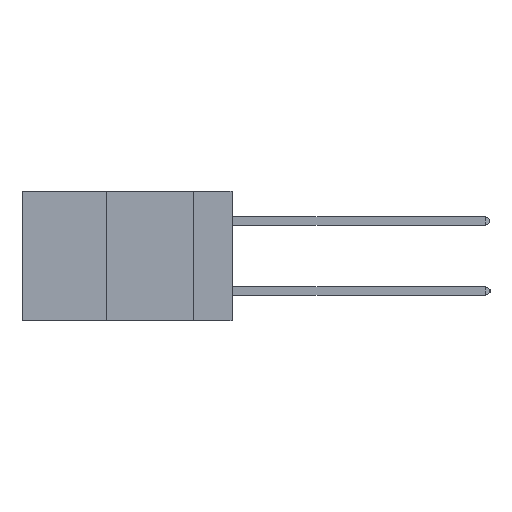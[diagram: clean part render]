
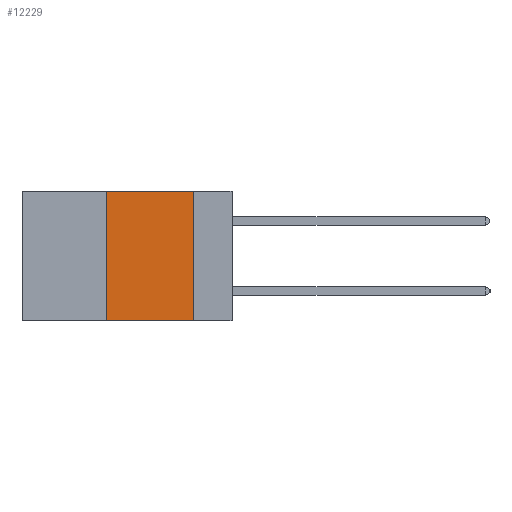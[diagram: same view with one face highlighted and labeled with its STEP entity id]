
A CAD part, left-side view. The second image highlights one B-rep face of the part: STEP entity #12229.
In plain terms, the highlighted planar face has unit normal (-1, 0, 0).
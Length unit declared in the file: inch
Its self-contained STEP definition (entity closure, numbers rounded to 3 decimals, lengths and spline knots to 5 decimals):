
#41 = LINE ( 'NONE', #6378, #4519 ) ;
#276 = VERTEX_POINT ( 'NONE', #10502 ) ;
#443 = VERTEX_POINT ( 'NONE', #11608 ) ;
#1178 = CARTESIAN_POINT ( 'NONE',  ( 0., 0.11, -0.37 ) ) ;
#2066 = CARTESIAN_POINT ( 'NONE',  ( 0., 0.36, 0. ) ) ;
#2390 = DIRECTION ( 'NONE',  ( 0., -1., 0. ) ) ;
#2874 = LINE ( 'NONE', #2066, #11031 ) ;
#3265 = VERTEX_POINT ( 'NONE', #1178 ) ;
#3268 = EDGE_CURVE ( 'NONE', #443, #276, #41, .T. ) ;
#3460 = AXIS2_PLACEMENT_3D ( 'NONE', #5574, #7523, #6670 ) ;
#4008 = EDGE_CURVE ( 'NONE', #11498, #443, #2874, .T. ) ;
#4235 = VECTOR ( 'NONE', #4794, 39.37008 ) ;
#4519 = VECTOR ( 'NONE', #2390, 39.37008 ) ;
#4695 = FACE_OUTER_BOUND ( 'NONE', #4941, .T. ) ;
#4794 = DIRECTION ( 'NONE',  ( 0., -1., 0. ) ) ;
#4941 = EDGE_LOOP ( 'NONE', ( #12663, #9753, #11478, #8268 ) ) ;
#5574 = CARTESIAN_POINT ( 'NONE',  ( 0., 0.6, 0. ) ) ;
#5943 = VECTOR ( 'NONE', #9829, 39.37008 ) ;
#6327 = DIRECTION ( 'NONE',  ( 0., 0., 1. ) ) ;
#6378 = CARTESIAN_POINT ( 'NONE',  ( 0., 0.6, 0. ) ) ;
#6670 = DIRECTION ( 'NONE',  ( 0., 0., -1. ) ) ;
#7146 = CARTESIAN_POINT ( 'NONE',  ( 0., 0.36, -0.37 ) ) ;
#7372 = EDGE_CURVE ( 'NONE', #11498, #3265, #11770, .T. ) ;
#7523 = DIRECTION ( 'NONE',  ( 1., 0., 0. ) ) ;
#7556 = LINE ( 'NONE', #11872, #5943 ) ;
#8268 = ORIENTED_EDGE ( 'NONE', *, *, #7372, .T. ) ;
#9353 = EDGE_CURVE ( 'NONE', #276, #3265, #7556, .T. ) ;
#9753 = ORIENTED_EDGE ( 'NONE', *, *, #3268, .F. ) ;
#9829 = DIRECTION ( 'NONE',  ( 0., 0., -1. ) ) ;
#10502 = CARTESIAN_POINT ( 'NONE',  ( 0., 0.11, 0. ) ) ;
#11031 = VECTOR ( 'NONE', #6327, 39.37008 ) ;
#11034 = CARTESIAN_POINT ( 'NONE',  ( 0., 0.6, -0.37 ) ) ;
#11478 = ORIENTED_EDGE ( 'NONE', *, *, #4008, .F. ) ;
#11498 = VERTEX_POINT ( 'NONE', #7146 ) ;
#11608 = CARTESIAN_POINT ( 'NONE',  ( 0., 0.36, 0. ) ) ;
#11770 = LINE ( 'NONE', #11034, #4235 ) ;
#11872 = CARTESIAN_POINT ( 'NONE',  ( 0., 0.11, 0. ) ) ;
#12229 = ADVANCED_FACE ( 'NONE', ( #4695 ), #12794, .F. ) ;
#12663 = ORIENTED_EDGE ( 'NONE', *, *, #9353, .F. ) ;
#12794 = PLANE ( 'NONE',  #3460 ) ;
